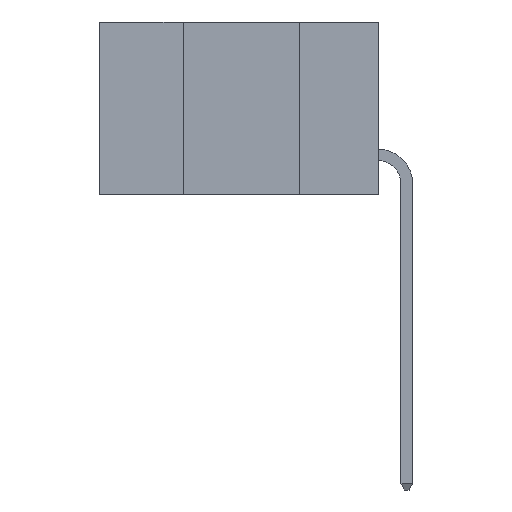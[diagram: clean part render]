
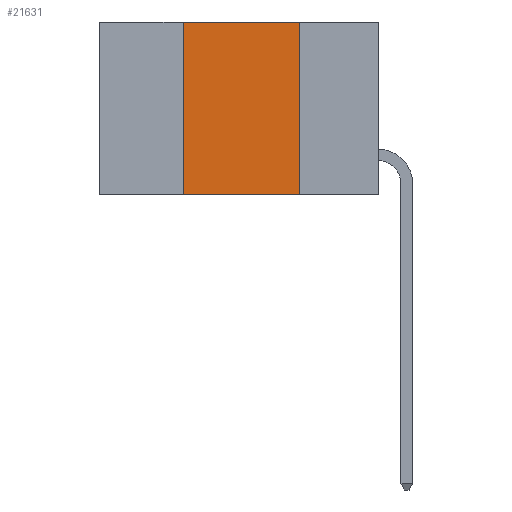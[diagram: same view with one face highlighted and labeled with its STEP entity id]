
A CAD part, left-side view. The second image highlights one B-rep face of the part: STEP entity #21631.
In plain terms, the highlighted planar face has unit normal (-1, 0, 0).
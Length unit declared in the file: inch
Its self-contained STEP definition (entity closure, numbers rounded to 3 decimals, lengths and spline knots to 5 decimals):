
#4460 = DIRECTION ( 'NONE',  ( 0., -1., 0. ) ) ;
#4540 = CARTESIAN_POINT ( 'NONE',  ( 0., 0.6, 0. ) ) ;
#4666 = CARTESIAN_POINT ( 'NONE',  ( 0., 0.17, 0. ) ) ;
#5457 = VECTOR ( 'NONE', #11535, 39.37008 ) ;
#5517 = CARTESIAN_POINT ( 'NONE',  ( 0., 0.6, 0. ) ) ;
#5646 = EDGE_CURVE ( 'NONE', #8329, #18842, #6290, .T. ) ;
#6290 = LINE ( 'NONE', #8620, #20461 ) ;
#6362 = DIRECTION ( 'NONE',  ( 0., 0., -1. ) ) ;
#7046 = EDGE_CURVE ( 'NONE', #12967, #18842, #8194, .T. ) ;
#8194 = LINE ( 'NONE', #20511, #12362 ) ;
#8329 = VERTEX_POINT ( 'NONE', #4666 ) ;
#8348 = EDGE_CURVE ( 'NONE', #17110, #8329, #17354, .T. ) ;
#8620 = CARTESIAN_POINT ( 'NONE',  ( 0., 0.17, -0.37 ) ) ;
#9073 = DIRECTION ( 'NONE',  ( 0., 0., -1. ) ) ;
#11535 = DIRECTION ( 'NONE',  ( 0., 0., 1. ) ) ;
#11972 = ORIENTED_EDGE ( 'NONE', *, *, #8348, .F. ) ;
#12362 = VECTOR ( 'NONE', #21382, 39.37008 ) ;
#12967 = VERTEX_POINT ( 'NONE', #16298 ) ;
#13197 = AXIS2_PLACEMENT_3D ( 'NONE', #4540, #17063, #6362 ) ;
#13697 = ORIENTED_EDGE ( 'NONE', *, *, #7046, .T. ) ;
#14004 = CARTESIAN_POINT ( 'NONE',  ( 0., 0.17, -0.37 ) ) ;
#15266 = PLANE ( 'NONE',  #13197 ) ;
#16199 = EDGE_LOOP ( 'NONE', ( #21339, #11972, #20554, #13697 ) ) ;
#16298 = CARTESIAN_POINT ( 'NONE',  ( 0., 0.42, -0.37 ) ) ;
#16794 = VECTOR ( 'NONE', #4460, 39.37008 ) ;
#17063 = DIRECTION ( 'NONE',  ( 1., 0., 0. ) ) ;
#17110 = VERTEX_POINT ( 'NONE', #22990 ) ;
#17354 = LINE ( 'NONE', #5517, #16794 ) ;
#17403 = EDGE_CURVE ( 'NONE', #12967, #17110, #18008, .T. ) ;
#18008 = LINE ( 'NONE', #22102, #5457 ) ;
#18842 = VERTEX_POINT ( 'NONE', #14004 ) ;
#20318 = FACE_OUTER_BOUND ( 'NONE', #16199, .T. ) ;
#20461 = VECTOR ( 'NONE', #9073, 39.37008 ) ;
#20511 = CARTESIAN_POINT ( 'NONE',  ( 0., 0.6, -0.37 ) ) ;
#20554 = ORIENTED_EDGE ( 'NONE', *, *, #17403, .F. ) ;
#21339 = ORIENTED_EDGE ( 'NONE', *, *, #5646, .F. ) ;
#21382 = DIRECTION ( 'NONE',  ( 0., -1., 0. ) ) ;
#21631 = ADVANCED_FACE ( 'NONE', ( #20318 ), #15266, .F. ) ;
#22102 = CARTESIAN_POINT ( 'NONE',  ( 0., 0.42, -0.37 ) ) ;
#22990 = CARTESIAN_POINT ( 'NONE',  ( 0., 0.42, 0. ) ) ;
